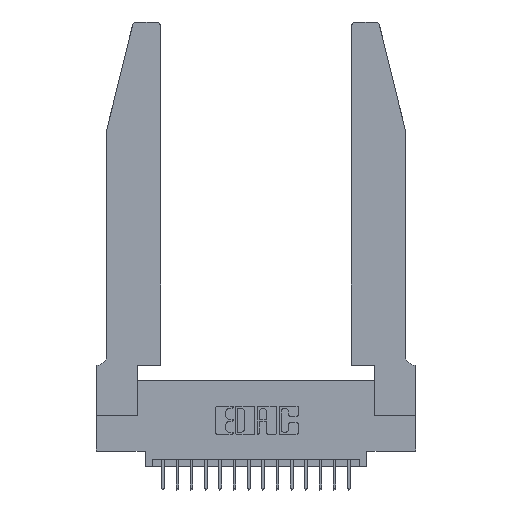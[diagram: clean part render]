
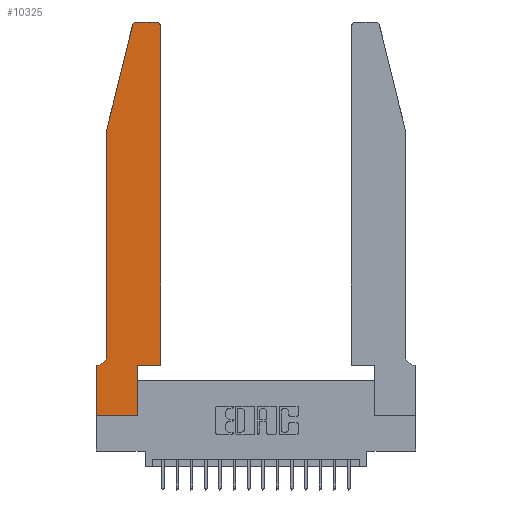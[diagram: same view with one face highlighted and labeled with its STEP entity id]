
A CAD part, top view. The second image highlights one B-rep face of the part: STEP entity #10325.
In plain terms, the highlighted planar face has unit normal (0, 0, 1).
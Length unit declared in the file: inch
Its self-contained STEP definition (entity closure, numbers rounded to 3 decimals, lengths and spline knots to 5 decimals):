
#73 = CARTESIAN_POINT ( 'NONE',  ( 0.0755, 0.42, 0.37 ) ) ;
#741 = DIRECTION ( 'NONE',  ( 1., 0., 0. ) ) ;
#907 = CARTESIAN_POINT ( 'NONE',  ( 0.284, 2.72, 0.37 ) ) ;
#1029 = LINE ( 'NONE', #1625, #2684 ) ;
#1257 = DIRECTION ( 'NONE',  ( 0., 1., 0. ) ) ;
#1374 = VERTEX_POINT ( 'NONE', #6105 ) ;
#1625 = CARTESIAN_POINT ( 'NONE',  ( 0., 0., 0.37 ) ) ;
#2179 = DIRECTION ( 'NONE',  ( 0., 0., 1. ) ) ;
#2372 = DIRECTION ( 'NONE',  ( 0., -1., 0. ) ) ;
#2607 = VERTEX_POINT ( 'NONE', #7606 ) ;
#2661 = LINE ( 'NONE', #13392, #17449 ) ;
#2684 = VECTOR ( 'NONE', #10754, 39.37008 ) ;
#2794 = LINE ( 'NONE', #19331, #6352 ) ;
#2897 = ORIENTED_EDGE ( 'NONE', *, *, #10933, .T. ) ;
#3021 = CARTESIAN_POINT ( 'NONE',  ( 0.0055, 0.35, 0.37 ) ) ;
#3106 = CARTESIAN_POINT ( 'NONE',  ( 0.0755, 2., 0.37 ) ) ;
#3130 = ORIENTED_EDGE ( 'NONE', *, *, #13806, .T. ) ;
#3184 = EDGE_CURVE ( 'NONE', #5988, #1374, #3365, .T. ) ;
#3365 = LINE ( 'NONE', #16428, #12695 ) ;
#3412 = EDGE_LOOP ( 'NONE', ( #17723, #9075, #14373, #3130, #19031, #15555, #9925, #19188, #7170, #2897, #6293, #5370 ) ) ;
#3683 = EDGE_CURVE ( 'NONE', #18434, #7814, #18602, .T. ) ;
#3931 = DIRECTION ( 'NONE',  ( 1., 0., 0. ) ) ;
#4353 = DIRECTION ( 'NONE',  ( -1., 0., 0. ) ) ;
#4360 = LINE ( 'NONE', #6894, #5057 ) ;
#4547 = DIRECTION ( 'NONE',  ( 1., 0., 0. ) ) ;
#4677 = VERTEX_POINT ( 'NONE', #12747 ) ;
#4736 = VECTOR ( 'NONE', #7933, 39.37008 ) ;
#4917 = CARTESIAN_POINT ( 'NONE',  ( 0.0755, 2., 0.37 ) ) ;
#5057 = VECTOR ( 'NONE', #2372, 39.37008 ) ;
#5299 = EDGE_CURVE ( 'NONE', #8922, #11330, #10940, .T. ) ;
#5370 = ORIENTED_EDGE ( 'NONE', *, *, #14575, .T. ) ;
#5576 = DIRECTION ( 'NONE',  ( -1., 0., 0. ) ) ;
#5694 = LINE ( 'NONE', #4917, #4736 ) ;
#5988 = VERTEX_POINT ( 'NONE', #13223 ) ;
#6105 = CARTESIAN_POINT ( 'NONE',  ( 0.2865, 0.35, 0.37 ) ) ;
#6293 = ORIENTED_EDGE ( 'NONE', *, *, #5299, .T. ) ;
#6299 = VERTEX_POINT ( 'NONE', #18584 ) ;
#6352 = VECTOR ( 'NONE', #5576, 39.37008 ) ;
#6893 = CARTESIAN_POINT ( 'NONE',  ( 0.4205, 2.72, 0.37 ) ) ;
#6894 = CARTESIAN_POINT ( 'NONE',  ( 0., 0., 0.37 ) ) ;
#7170 = ORIENTED_EDGE ( 'NONE', *, *, #3184, .T. ) ;
#7312 = CARTESIAN_POINT ( 'NONE',  ( 0.4505, 0.35, 0.37 ) ) ;
#7606 = CARTESIAN_POINT ( 'NONE',  ( 0.0755, 2., 0.37 ) ) ;
#7814 = VERTEX_POINT ( 'NONE', #12214 ) ;
#7819 = CARTESIAN_POINT ( 'NONE',  ( 0., 0.35, 0.37 ) ) ;
#7933 = DIRECTION ( 'NONE',  ( 0., -1., 0. ) ) ;
#8314 = VECTOR ( 'NONE', #13184, 39.37008 ) ;
#8524 = AXIS2_PLACEMENT_3D ( 'NONE', #18029, #13315, #13443 ) ;
#8628 = CARTESIAN_POINT ( 'NONE',  ( 0.4505, 0.35, 0.37 ) ) ;
#8922 = VERTEX_POINT ( 'NONE', #8944 ) ;
#8944 = CARTESIAN_POINT ( 'NONE',  ( 0.4505, 0.35, 0.37 ) ) ;
#9075 = ORIENTED_EDGE ( 'NONE', *, *, #3683, .T. ) ;
#9132 = VECTOR ( 'NONE', #16639, 39.37008 ) ;
#9700 = EDGE_CURVE ( 'NONE', #7814, #2607, #18883, .T. ) ;
#9925 = ORIENTED_EDGE ( 'NONE', *, *, #12046, .T. ) ;
#10325 = ADVANCED_FACE ( 'NONE', ( #13539 ), #15171, .T. ) ;
#10694 = CIRCLE ( 'NONE', #8524, 0.07 ) ;
#10754 = DIRECTION ( 'NONE',  ( 1., 0., 0. ) ) ;
#10933 = EDGE_CURVE ( 'NONE', #1374, #8922, #11593, .T. ) ;
#10940 = LINE ( 'NONE', #8628, #8314 ) ;
#11330 = VERTEX_POINT ( 'NONE', #18668 ) ;
#11593 = LINE ( 'NONE', #7312, #18266 ) ;
#12046 = EDGE_CURVE ( 'NONE', #6299, #4677, #4360, .T. ) ;
#12214 = CARTESIAN_POINT ( 'NONE',  ( 0.25487, 2.72718, 0.37 ) ) ;
#12445 = VERTEX_POINT ( 'NONE', #3021 ) ;
#12695 = VECTOR ( 'NONE', #1257, 39.37008 ) ;
#12747 = CARTESIAN_POINT ( 'NONE',  ( 0., 0., 0.37 ) ) ;
#12939 = EDGE_CURVE ( 'NONE', #17025, #18434, #2661, .T. ) ;
#13184 = DIRECTION ( 'NONE',  ( 0., 1., 0. ) ) ;
#13223 = CARTESIAN_POINT ( 'NONE',  ( 0.2865, 0., 0.37 ) ) ;
#13241 = DIRECTION ( 'NONE',  ( 0., 0., 1. ) ) ;
#13315 = DIRECTION ( 'NONE',  ( 0., 0., -1. ) ) ;
#13392 = CARTESIAN_POINT ( 'NONE',  ( 0.2605, 2.75, 0.37 ) ) ;
#13443 = DIRECTION ( 'NONE',  ( -1., 0., 0. ) ) ;
#13539 = FACE_OUTER_BOUND ( 'NONE', #3412, .T. ) ;
#13806 = EDGE_CURVE ( 'NONE', #2607, #18239, #5694, .T. ) ;
#13854 = DIRECTION ( 'NONE',  ( 0., 0., 1. ) ) ;
#14018 = CARTESIAN_POINT ( 'NONE',  ( 0.284, 2.75, 0.37 ) ) ;
#14373 = ORIENTED_EDGE ( 'NONE', *, *, #9700, .T. ) ;
#14575 = EDGE_CURVE ( 'NONE', #11330, #17025, #18324, .T. ) ;
#15171 = PLANE ( 'NONE',  #15618 ) ;
#15327 = EDGE_CURVE ( 'NONE', #12445, #6299, #2794, .T. ) ;
#15430 = EDGE_CURVE ( 'NONE', #18239, #12445, #10694, .T. ) ;
#15555 = ORIENTED_EDGE ( 'NONE', *, *, #15327, .T. ) ;
#15618 = AXIS2_PLACEMENT_3D ( 'NONE', #7819, #13854, #4547 ) ;
#16026 = CARTESIAN_POINT ( 'NONE',  ( 0.4205, 2.75, 0.37 ) ) ;
#16428 = CARTESIAN_POINT ( 'NONE',  ( 0.2865, 0.35, 0.37 ) ) ;
#16597 = DIRECTION ( 'NONE',  ( 1., 0., 0. ) ) ;
#16639 = DIRECTION ( 'NONE',  ( -0.239, -0.971, 0. ) ) ;
#17025 = VERTEX_POINT ( 'NONE', #16026 ) ;
#17064 = AXIS2_PLACEMENT_3D ( 'NONE', #6893, #2179, #741 ) ;
#17449 = VECTOR ( 'NONE', #4353, 39.37008 ) ;
#17723 = ORIENTED_EDGE ( 'NONE', *, *, #12939, .T. ) ;
#18029 = CARTESIAN_POINT ( 'NONE',  ( 0.0055, 0.42, 0.37 ) ) ;
#18239 = VERTEX_POINT ( 'NONE', #73 ) ;
#18266 = VECTOR ( 'NONE', #16597, 39.37008 ) ;
#18324 = CIRCLE ( 'NONE', #17064, 0.03 ) ;
#18434 = VERTEX_POINT ( 'NONE', #14018 ) ;
#18437 = EDGE_CURVE ( 'NONE', #4677, #5988, #1029, .T. ) ;
#18584 = CARTESIAN_POINT ( 'NONE',  ( 0., 0.35, 0.37 ) ) ;
#18602 = CIRCLE ( 'NONE', #19076, 0.03 ) ;
#18668 = CARTESIAN_POINT ( 'NONE',  ( 0.4505, 2.72, 0.37 ) ) ;
#18883 = LINE ( 'NONE', #3106, #9132 ) ;
#19031 = ORIENTED_EDGE ( 'NONE', *, *, #15430, .T. ) ;
#19076 = AXIS2_PLACEMENT_3D ( 'NONE', #907, #13241, #3931 ) ;
#19188 = ORIENTED_EDGE ( 'NONE', *, *, #18437, .T. ) ;
#19331 = CARTESIAN_POINT ( 'NONE',  ( 0.0755, 0.35, 0.37 ) ) ;
